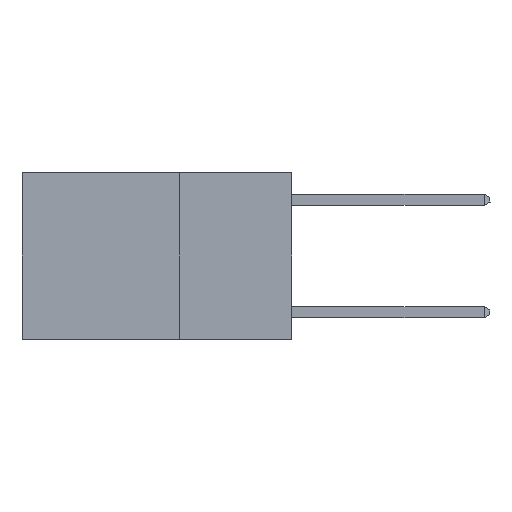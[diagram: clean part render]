
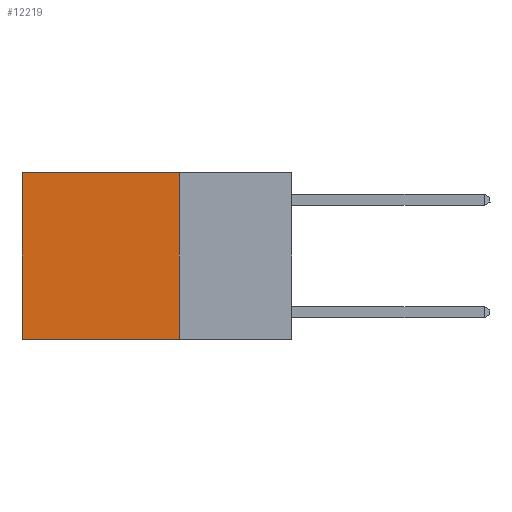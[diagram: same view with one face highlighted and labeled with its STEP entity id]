
A CAD part, left-side view. The second image highlights one B-rep face of the part: STEP entity #12219.
In plain terms, the highlighted planar face has unit normal (-1, 0, 0).
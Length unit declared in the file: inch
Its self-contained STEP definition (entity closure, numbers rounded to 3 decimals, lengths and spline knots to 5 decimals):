
#654 = FACE_OUTER_BOUND ( 'NONE', #16235, .T. ) ;
#792 = CARTESIAN_POINT ( 'NONE',  ( 0.2625, 0.6, 0. ) ) ;
#1587 = VERTEX_POINT ( 'NONE', #15237 ) ;
#1695 = VECTOR ( 'NONE', #8600, 39.37008 ) ;
#2214 = VERTEX_POINT ( 'NONE', #14218 ) ;
#2736 = ORIENTED_EDGE ( 'NONE', *, *, #7994, .T. ) ;
#3130 = DIRECTION ( 'NONE',  ( 0., 0., -1. ) ) ;
#4681 = AXIS2_PLACEMENT_3D ( 'NONE', #9438, #6878, #15851 ) ;
#5388 = EDGE_CURVE ( 'NONE', #7793, #2214, #8581, .T. ) ;
#5689 = DIRECTION ( 'NONE',  ( 0., 1., 0. ) ) ;
#6878 = DIRECTION ( 'NONE',  ( 1., 0., 0. ) ) ;
#7461 = ORIENTED_EDGE ( 'NONE', *, *, #12297, .F. ) ;
#7793 = VERTEX_POINT ( 'NONE', #9343 ) ;
#7994 = EDGE_CURVE ( 'NONE', #7793, #1587, #13602, .T. ) ;
#8196 = VECTOR ( 'NONE', #3130, 39.37008 ) ;
#8401 = DIRECTION ( 'NONE',  ( 0., 1., 0. ) ) ;
#8581 = LINE ( 'NONE', #10907, #8196 ) ;
#8600 = DIRECTION ( 'NONE',  ( 0., 0., -1. ) ) ;
#8625 = LINE ( 'NONE', #792, #1695 ) ;
#8857 = VERTEX_POINT ( 'NONE', #10813 ) ;
#9343 = CARTESIAN_POINT ( 'NONE',  ( 0.2625, 0.25, 0. ) ) ;
#9438 = CARTESIAN_POINT ( 'NONE',  ( 0.2625, 0.25, 0. ) ) ;
#9831 = VECTOR ( 'NONE', #5689, 39.37008 ) ;
#10813 = CARTESIAN_POINT ( 'NONE',  ( 0.2625, 0.6, -0.37 ) ) ;
#10907 = CARTESIAN_POINT ( 'NONE',  ( 0.2625, 0.25, 0. ) ) ;
#10920 = EDGE_CURVE ( 'NONE', #1587, #8857, #8625, .T. ) ;
#11001 = CARTESIAN_POINT ( 'NONE',  ( 0.2625, 0.25, 0. ) ) ;
#12219 = ADVANCED_FACE ( 'NONE', ( #654 ), #14601, .F. ) ;
#12297 = EDGE_CURVE ( 'NONE', #2214, #8857, #13319, .T. ) ;
#13319 = LINE ( 'NONE', #14707, #9831 ) ;
#13602 = LINE ( 'NONE', #11001, #16489 ) ;
#14218 = CARTESIAN_POINT ( 'NONE',  ( 0.2625, 0.25, -0.37 ) ) ;
#14547 = ORIENTED_EDGE ( 'NONE', *, *, #10920, .T. ) ;
#14601 = PLANE ( 'NONE',  #4681 ) ;
#14707 = CARTESIAN_POINT ( 'NONE',  ( 0.2625, 0.25, -0.37 ) ) ;
#14818 = ORIENTED_EDGE ( 'NONE', *, *, #5388, .F. ) ;
#15237 = CARTESIAN_POINT ( 'NONE',  ( 0.2625, 0.6, 0. ) ) ;
#15851 = DIRECTION ( 'NONE',  ( 0., 0., -1. ) ) ;
#16235 = EDGE_LOOP ( 'NONE', ( #14547, #7461, #14818, #2736 ) ) ;
#16489 = VECTOR ( 'NONE', #8401, 39.37008 ) ;
